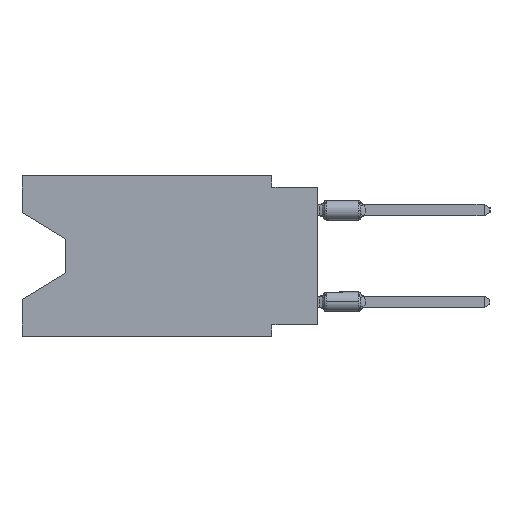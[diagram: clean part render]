
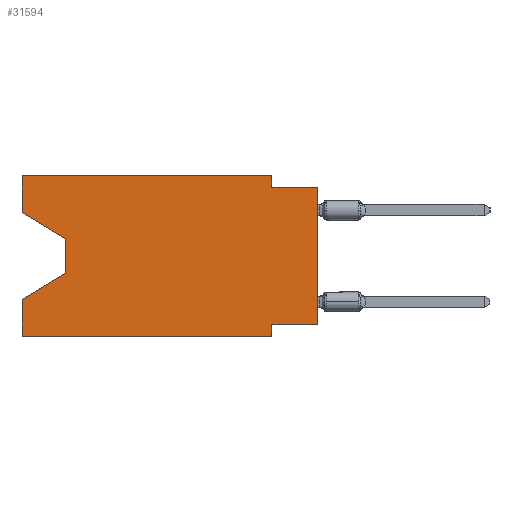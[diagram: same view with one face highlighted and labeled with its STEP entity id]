
A CAD part, left-side view. The second image highlights one B-rep face of the part: STEP entity #31594.
In plain terms, the highlighted planar face has unit normal (-1, 0, 0).
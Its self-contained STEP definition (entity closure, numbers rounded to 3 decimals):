
#16 = EDGE_CURVE ( 'NONE', #22028, #28172, #8430, .T. ) ;
#19 = VECTOR ( 'NONE', #11986, 1000. ) ;
#156 = VECTOR ( 'NONE', #4313, 1000. ) ;
#435 = CARTESIAN_POINT ( 'NONE',  ( 0., 0., -0.635 ) ) ;
#1181 = CARTESIAN_POINT ( 'NONE',  ( 0., 16.383, 0. ) ) ;
#2077 = LINE ( 'NONE', #24813, #19724 ) ;
#2113 = CARTESIAN_POINT ( 'NONE',  ( 0., 13.97, -5.385 ) ) ;
#2212 = EDGE_CURVE ( 'NONE', #18948, #24209, #2077, .T. ) ;
#2611 = LINE ( 'NONE', #435, #32362 ) ;
#3197 = EDGE_CURVE ( 'NONE', #29636, #9756, #2611, .T. ) ;
#3814 = VECTOR ( 'NONE', #31134, 1000. ) ;
#3881 = VECTOR ( 'NONE', #22985, 1000. ) ;
#4313 = DIRECTION ( 'NONE',  ( 0., 0., 1. ) ) ;
#4685 = CARTESIAN_POINT ( 'NONE',  ( 0., 2.54, -8.89 ) ) ;
#5152 = ORIENTED_EDGE ( 'NONE', *, *, #7866, .F. ) ;
#6253 = CARTESIAN_POINT ( 'NONE',  ( 0., 13.97, -5.385 ) ) ;
#6310 = ORIENTED_EDGE ( 'NONE', *, *, #26466, .F. ) ;
#6583 = VERTEX_POINT ( 'NONE', #25674 ) ;
#7366 = ORIENTED_EDGE ( 'NONE', *, *, #2212, .T. ) ;
#7828 = CARTESIAN_POINT ( 'NONE',  ( 0., 16.383, 0. ) ) ;
#7866 = EDGE_CURVE ( 'NONE', #18948, #20737, #11981, .T. ) ;
#8430 = LINE ( 'NONE', #21107, #27041 ) ;
#8788 = ORIENTED_EDGE ( 'NONE', *, *, #23378, .T. ) ;
#8792 = CARTESIAN_POINT ( 'NONE',  ( 0., 16.383, 0. ) ) ;
#9604 = CARTESIAN_POINT ( 'NONE',  ( 0., 0., 0. ) ) ;
#9627 = ORIENTED_EDGE ( 'NONE', *, *, #3197, .F. ) ;
#9639 = LINE ( 'NONE', #4685, #26731 ) ;
#9756 = VERTEX_POINT ( 'NONE', #31829 ) ;
#9815 = DIRECTION ( 'NONE',  ( 0., 0., -1. ) ) ;
#9973 = DIRECTION ( 'NONE',  ( 1., 0., 0. ) ) ;
#10041 = VERTEX_POINT ( 'NONE', #6253 ) ;
#10627 = VERTEX_POINT ( 'NONE', #17734 ) ;
#11381 = CARTESIAN_POINT ( 'NONE',  ( 0., 2.54, -8.255 ) ) ;
#11396 = ORIENTED_EDGE ( 'NONE', *, *, #23194, .F. ) ;
#11493 = LINE ( 'NONE', #32085, #19 ) ;
#11783 = EDGE_CURVE ( 'NONE', #24209, #10041, #11493, .T. ) ;
#11981 = LINE ( 'NONE', #16435, #25500 ) ;
#11986 = DIRECTION ( 'NONE',  ( 0., 0., -1. ) ) ;
#12517 = CARTESIAN_POINT ( 'NONE',  ( 0., 2.54, 0. ) ) ;
#12680 = LINE ( 'NONE', #12517, #3814 ) ;
#12924 = LINE ( 'NONE', #28087, #3881 ) ;
#14751 = FACE_OUTER_BOUND ( 'NONE', #17824, .T. ) ;
#15227 = AXIS2_PLACEMENT_3D ( 'NONE', #7828, #9973, #9815 ) ;
#15229 = EDGE_CURVE ( 'NONE', #6583, #29636, #12680, .T. ) ;
#15650 = ORIENTED_EDGE ( 'NONE', *, *, #16, .F. ) ;
#15843 = DIRECTION ( 'NONE',  ( 0., 1., 0. ) ) ;
#16435 = CARTESIAN_POINT ( 'NONE',  ( 0., 16.383, 0. ) ) ;
#16840 = CARTESIAN_POINT ( 'NONE',  ( 0., 16.383, 0. ) ) ;
#16891 = ORIENTED_EDGE ( 'NONE', *, *, #28622, .T. ) ;
#17734 = CARTESIAN_POINT ( 'NONE',  ( 0., 16.383, -8.89 ) ) ;
#17824 = EDGE_LOOP ( 'NONE', ( #7366, #18256, #16891, #6310, #8788, #11396, #15650, #26795, #9627, #26639, #22862, #5152 ) ) ;
#18063 = DIRECTION ( 'NONE',  ( 0., -1., 0. ) ) ;
#18256 = ORIENTED_EDGE ( 'NONE', *, *, #11783, .T. ) ;
#18534 = VERTEX_POINT ( 'NONE', #25826 ) ;
#18816 = DIRECTION ( 'NONE',  ( 0., -1., 0. ) ) ;
#18948 = VERTEX_POINT ( 'NONE', #25792 ) ;
#19724 = VECTOR ( 'NONE', #21668, 1000. ) ;
#20737 = VERTEX_POINT ( 'NONE', #1181 ) ;
#21107 = CARTESIAN_POINT ( 'NONE',  ( 0., 0., -8.255 ) ) ;
#21379 = CARTESIAN_POINT ( 'NONE',  ( 0., 2.54, -0.635 ) ) ;
#21668 = DIRECTION ( 'NONE',  ( 0., -0.855, -0.519 ) ) ;
#22028 = VERTEX_POINT ( 'NONE', #30033 ) ;
#22285 = DIRECTION ( 'NONE',  ( 0., 0., 1. ) ) ;
#22377 = DIRECTION ( 'NONE',  ( 0., 0.855, -0.519 ) ) ;
#22862 = ORIENTED_EDGE ( 'NONE', *, *, #30666, .F. ) ;
#22985 = DIRECTION ( 'NONE',  ( 0., -1., 0. ) ) ;
#23027 = CARTESIAN_POINT ( 'NONE',  ( 0., 13.97, -3.505 ) ) ;
#23194 = EDGE_CURVE ( 'NONE', #28172, #24936, #9639, .T. ) ;
#23378 = EDGE_CURVE ( 'NONE', #10627, #24936, #12924, .T. ) ;
#23447 = LINE ( 'NONE', #16840, #156 ) ;
#24152 = DIRECTION ( 'NONE',  ( 0., 0., -1. ) ) ;
#24209 = VERTEX_POINT ( 'NONE', #23027 ) ;
#24813 = CARTESIAN_POINT ( 'NONE',  ( 0., 16.383, -2.038 ) ) ;
#24936 = VERTEX_POINT ( 'NONE', #29079 ) ;
#25500 = VECTOR ( 'NONE', #32079, 1000. ) ;
#25673 = VECTOR ( 'NONE', #22377, 1000. ) ;
#25674 = CARTESIAN_POINT ( 'NONE',  ( 0., 2.54, 0. ) ) ;
#25792 = CARTESIAN_POINT ( 'NONE',  ( 0., 16.383, -2.038 ) ) ;
#25826 = CARTESIAN_POINT ( 'NONE',  ( 0., 16.383, -6.852 ) ) ;
#26466 = EDGE_CURVE ( 'NONE', #10627, #18534, #23447, .T. ) ;
#26639 = ORIENTED_EDGE ( 'NONE', *, *, #15229, .F. ) ;
#26731 = VECTOR ( 'NONE', #24152, 1000. ) ;
#26795 = ORIENTED_EDGE ( 'NONE', *, *, #30775, .T. ) ;
#27041 = VECTOR ( 'NONE', #15843, 1000. ) ;
#27605 = PLANE ( 'NONE',  #15227 ) ;
#28087 = CARTESIAN_POINT ( 'NONE',  ( 0., 16.383, -8.89 ) ) ;
#28172 = VERTEX_POINT ( 'NONE', #11381 ) ;
#28622 = EDGE_CURVE ( 'NONE', #10041, #18534, #32098, .T. ) ;
#28893 = VECTOR ( 'NONE', #22285, 1000. ) ;
#29079 = CARTESIAN_POINT ( 'NONE',  ( 0., 2.54, -8.89 ) ) ;
#29636 = VERTEX_POINT ( 'NONE', #21379 ) ;
#30033 = CARTESIAN_POINT ( 'NONE',  ( 0., 0., -8.255 ) ) ;
#30460 = VECTOR ( 'NONE', #18816, 1000. ) ;
#30666 = EDGE_CURVE ( 'NONE', #20737, #6583, #31681, .T. ) ;
#30775 = EDGE_CURVE ( 'NONE', #22028, #9756, #32170, .T. ) ;
#31134 = DIRECTION ( 'NONE',  ( 0., 0., -1. ) ) ;
#31594 = ADVANCED_FACE ( 'NONE', ( #14751 ), #27605, .F. ) ;
#31681 = LINE ( 'NONE', #8792, #30460 ) ;
#31829 = CARTESIAN_POINT ( 'NONE',  ( 0., 0., -0.635 ) ) ;
#32079 = DIRECTION ( 'NONE',  ( 0., 0., 1. ) ) ;
#32085 = CARTESIAN_POINT ( 'NONE',  ( 0., 13.97, -3.505 ) ) ;
#32098 = LINE ( 'NONE', #2113, #25673 ) ;
#32170 = LINE ( 'NONE', #9604, #28893 ) ;
#32362 = VECTOR ( 'NONE', #18063, 1000. ) ;
